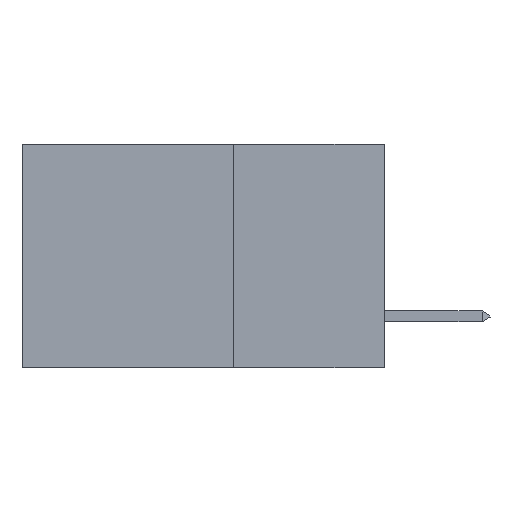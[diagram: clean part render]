
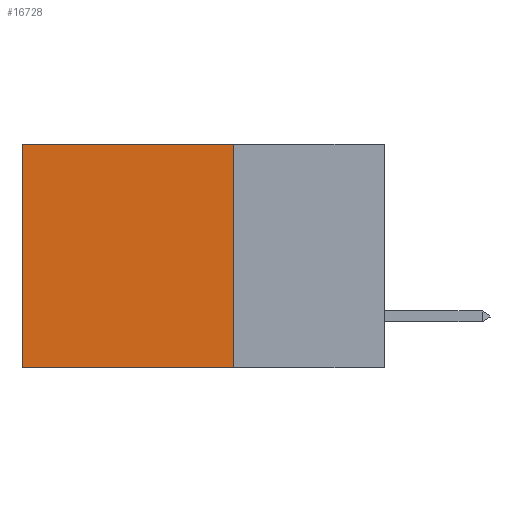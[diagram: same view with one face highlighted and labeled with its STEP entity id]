
A CAD part, left-side view. The second image highlights one B-rep face of the part: STEP entity #16728.
In plain terms, the highlighted planar face has unit normal (-1, 0, 0).
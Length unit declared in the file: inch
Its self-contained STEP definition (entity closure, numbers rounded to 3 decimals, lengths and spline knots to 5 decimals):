
#1498 = ORIENTED_EDGE ( 'NONE', *, *, #35841, .T. ) ;
#3796 = VECTOR ( 'NONE', #5476, 39.37008 ) ;
#4855 = LINE ( 'NONE', #38334, #3796 ) ;
#5077 = EDGE_CURVE ( 'NONE', #32940, #14306, #28761, .T. ) ;
#5421 = CARTESIAN_POINT ( 'NONE',  ( 0.2875, 0.25, 0. ) ) ;
#5476 = DIRECTION ( 'NONE',  ( 0., 1., 0. ) ) ;
#5983 = EDGE_LOOP ( 'NONE', ( #7162, #36505, #27185, #1498 ) ) ;
#7162 = ORIENTED_EDGE ( 'NONE', *, *, #5077, .T. ) ;
#10077 = CARTESIAN_POINT ( 'NONE',  ( 0.2875, 0.25, -0.37 ) ) ;
#11836 = VERTEX_POINT ( 'NONE', #33509 ) ;
#11848 = FACE_OUTER_BOUND ( 'NONE', #5983, .T. ) ;
#12964 = LINE ( 'NONE', #5421, #26330 ) ;
#14306 = VERTEX_POINT ( 'NONE', #21902 ) ;
#15296 = EDGE_CURVE ( 'NONE', #11836, #31734, #12964, .T. ) ;
#15807 = DIRECTION ( 'NONE',  ( 0., 0., -1. ) ) ;
#15850 = VECTOR ( 'NONE', #39207, 39.37008 ) ;
#16728 = ADVANCED_FACE ( 'NONE', ( #11848 ), #29642, .F. ) ;
#19516 = CARTESIAN_POINT ( 'NONE',  ( 0.2875, 0.25, 0. ) ) ;
#20817 = EDGE_CURVE ( 'NONE', #31734, #14306, #26277, .T. ) ;
#21902 = CARTESIAN_POINT ( 'NONE',  ( 0.2875, 0.6, -0.37 ) ) ;
#24251 = AXIS2_PLACEMENT_3D ( 'NONE', #19516, #26287, #15807 ) ;
#25921 = CARTESIAN_POINT ( 'NONE',  ( 0.2875, 0.6, 0. ) ) ;
#26277 = LINE ( 'NONE', #10077, #37601 ) ;
#26287 = DIRECTION ( 'NONE',  ( 1., 0., 0. ) ) ;
#26330 = VECTOR ( 'NONE', #37352, 39.37008 ) ;
#27185 = ORIENTED_EDGE ( 'NONE', *, *, #15296, .F. ) ;
#27602 = DIRECTION ( 'NONE',  ( 0., 1., 0. ) ) ;
#28761 = LINE ( 'NONE', #25921, #15850 ) ;
#29642 = PLANE ( 'NONE',  #24251 ) ;
#31734 = VERTEX_POINT ( 'NONE', #32582 ) ;
#32582 = CARTESIAN_POINT ( 'NONE',  ( 0.2875, 0.25, -0.37 ) ) ;
#32940 = VERTEX_POINT ( 'NONE', #41807 ) ;
#33509 = CARTESIAN_POINT ( 'NONE',  ( 0.2875, 0.25, 0. ) ) ;
#35841 = EDGE_CURVE ( 'NONE', #11836, #32940, #4855, .T. ) ;
#36505 = ORIENTED_EDGE ( 'NONE', *, *, #20817, .F. ) ;
#37352 = DIRECTION ( 'NONE',  ( 0., 0., -1. ) ) ;
#37601 = VECTOR ( 'NONE', #27602, 39.37008 ) ;
#38334 = CARTESIAN_POINT ( 'NONE',  ( 0.2875, 0.25, 0. ) ) ;
#39207 = DIRECTION ( 'NONE',  ( 0., 0., -1. ) ) ;
#41807 = CARTESIAN_POINT ( 'NONE',  ( 0.2875, 0.6, 0. ) ) ;
